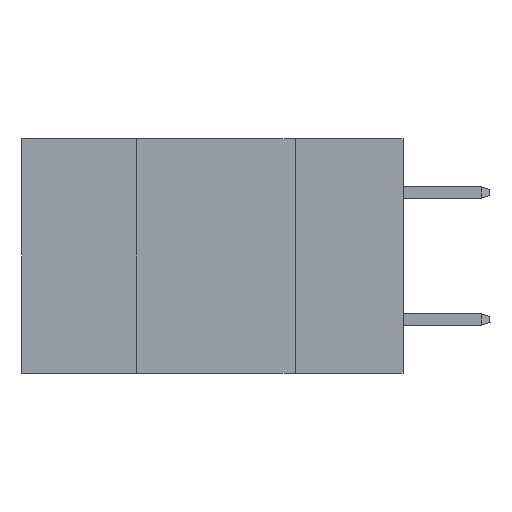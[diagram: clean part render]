
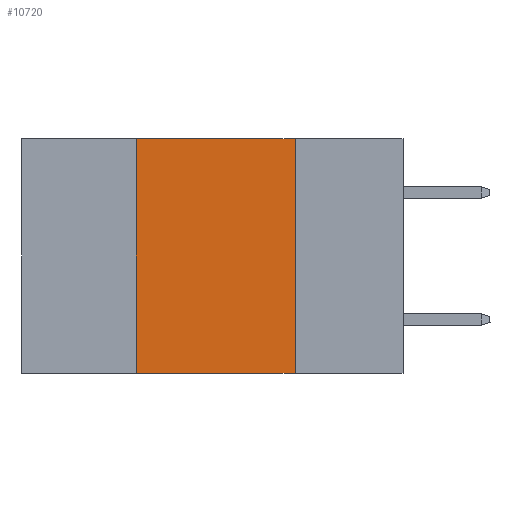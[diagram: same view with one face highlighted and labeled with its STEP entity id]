
A CAD part, left-side view. The second image highlights one B-rep face of the part: STEP entity #10720.
In plain terms, the highlighted planar face has unit normal (-1, 0, 0).
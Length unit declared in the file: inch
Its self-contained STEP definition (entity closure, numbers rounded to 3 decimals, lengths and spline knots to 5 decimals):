
#355 = DIRECTION ( 'NONE',  ( 0., -1., 0. ) ) ;
#716 = CARTESIAN_POINT ( 'NONE',  ( 0., 0.17, -0.37 ) ) ;
#1205 = AXIS2_PLACEMENT_3D ( 'NONE', #10873, #2416, #1346 ) ;
#1346 = DIRECTION ( 'NONE',  ( 0., 0., -1. ) ) ;
#1383 = LINE ( 'NONE', #8263, #3371 ) ;
#1672 = DIRECTION ( 'NONE',  ( 0., -1., 0. ) ) ;
#2060 = DIRECTION ( 'NONE',  ( 0., 0., -1. ) ) ;
#2416 = DIRECTION ( 'NONE',  ( 1., 0., 0. ) ) ;
#2797 = EDGE_CURVE ( 'NONE', #4308, #6717, #3928, .T. ) ;
#2857 = CARTESIAN_POINT ( 'NONE',  ( 0., 0.6, -0.37 ) ) ;
#2998 = LINE ( 'NONE', #10636, #10790 ) ;
#3217 = ORIENTED_EDGE ( 'NONE', *, *, #4807, .F. ) ;
#3371 = VECTOR ( 'NONE', #4192, 39.37008 ) ;
#3850 = LINE ( 'NONE', #2857, #7055 ) ;
#3857 = EDGE_CURVE ( 'NONE', #4647, #4308, #2998, .T. ) ;
#3928 = LINE ( 'NONE', #8825, #6949 ) ;
#4192 = DIRECTION ( 'NONE',  ( 0., 0., 1. ) ) ;
#4308 = VERTEX_POINT ( 'NONE', #5495 ) ;
#4647 = VERTEX_POINT ( 'NONE', #11571 ) ;
#4807 = EDGE_CURVE ( 'NONE', #7105, #4647, #1383, .T. ) ;
#5495 = CARTESIAN_POINT ( 'NONE',  ( 0., 0.17, 0. ) ) ;
#6344 = EDGE_LOOP ( 'NONE', ( #6832, #7777, #3217, #10530 ) ) ;
#6717 = VERTEX_POINT ( 'NONE', #716 ) ;
#6832 = ORIENTED_EDGE ( 'NONE', *, *, #2797, .F. ) ;
#6949 = VECTOR ( 'NONE', #2060, 39.37008 ) ;
#7023 = FACE_OUTER_BOUND ( 'NONE', #6344, .T. ) ;
#7055 = VECTOR ( 'NONE', #1672, 39.37008 ) ;
#7105 = VERTEX_POINT ( 'NONE', #9024 ) ;
#7611 = EDGE_CURVE ( 'NONE', #7105, #6717, #3850, .T. ) ;
#7777 = ORIENTED_EDGE ( 'NONE', *, *, #3857, .F. ) ;
#8263 = CARTESIAN_POINT ( 'NONE',  ( 0., 0.42, 0. ) ) ;
#8825 = CARTESIAN_POINT ( 'NONE',  ( 0., 0.17, 0. ) ) ;
#9024 = CARTESIAN_POINT ( 'NONE',  ( 0., 0.42, -0.37 ) ) ;
#10530 = ORIENTED_EDGE ( 'NONE', *, *, #7611, .T. ) ;
#10636 = CARTESIAN_POINT ( 'NONE',  ( 0., 0.6, 0. ) ) ;
#10720 = ADVANCED_FACE ( 'NONE', ( #7023 ), #11925, .F. ) ;
#10790 = VECTOR ( 'NONE', #355, 39.37008 ) ;
#10873 = CARTESIAN_POINT ( 'NONE',  ( 0., 0.6, 0. ) ) ;
#11571 = CARTESIAN_POINT ( 'NONE',  ( 0., 0.42, 0. ) ) ;
#11925 = PLANE ( 'NONE',  #1205 ) ;
